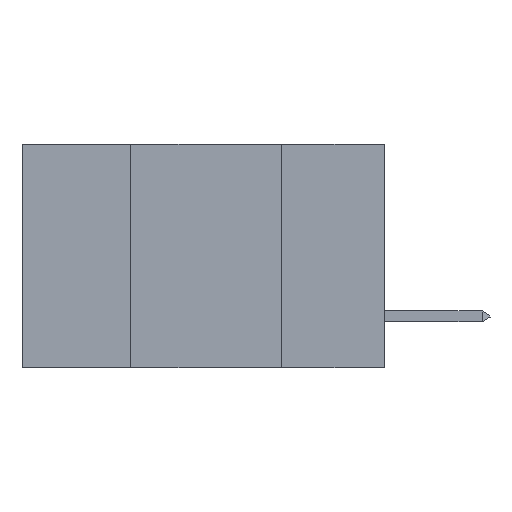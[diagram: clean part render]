
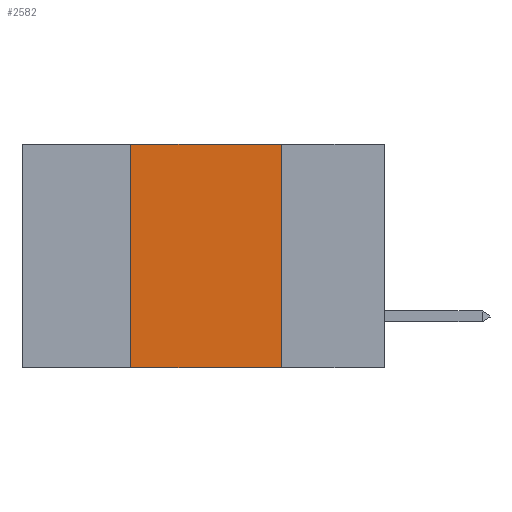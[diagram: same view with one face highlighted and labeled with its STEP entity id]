
A CAD part, left-side view. The second image highlights one B-rep face of the part: STEP entity #2582.
In plain terms, the highlighted planar face has unit normal (-1, 0, 0).
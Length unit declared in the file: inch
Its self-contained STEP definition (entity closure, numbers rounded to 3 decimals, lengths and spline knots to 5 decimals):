
#131 = LINE ( 'NONE', #482, #4072 ) ;
#385 = VERTEX_POINT ( 'NONE', #13871 ) ;
#482 = CARTESIAN_POINT ( 'NONE',  ( 0., 0.6, -0.37 ) ) ;
#1305 = DIRECTION ( 'NONE',  ( 0., -1., 0. ) ) ;
#2582 = ADVANCED_FACE ( 'NONE', ( #24983 ), #10530, .F. ) ;
#3062 = VERTEX_POINT ( 'NONE', #8569 ) ;
#4072 = VECTOR ( 'NONE', #21789, 39.37008 ) ;
#4646 = DIRECTION ( 'NONE',  ( 1., 0., 0. ) ) ;
#4726 = EDGE_CURVE ( 'NONE', #7918, #3062, #7692, .T. ) ;
#6712 = DIRECTION ( 'NONE',  ( 0., 0., -1. ) ) ;
#7692 = LINE ( 'NONE', #21678, #22477 ) ;
#7867 = LINE ( 'NONE', #24668, #24115 ) ;
#7918 = VERTEX_POINT ( 'NONE', #24495 ) ;
#8342 = ORIENTED_EDGE ( 'NONE', *, *, #4726, .F. ) ;
#8569 = CARTESIAN_POINT ( 'NONE',  ( 0., 0.42, 0. ) ) ;
#9111 = VERTEX_POINT ( 'NONE', #10108 ) ;
#10108 = CARTESIAN_POINT ( 'NONE',  ( 0., 0.17, -0.37 ) ) ;
#10530 = PLANE ( 'NONE',  #23315 ) ;
#11037 = VECTOR ( 'NONE', #15741, 39.37008 ) ;
#12194 = DIRECTION ( 'NONE',  ( 0., 0., 1. ) ) ;
#13707 = EDGE_LOOP ( 'NONE', ( #16742, #18024, #8342, #19715 ) ) ;
#13871 = CARTESIAN_POINT ( 'NONE',  ( 0., 0.17, 0. ) ) ;
#14305 = CARTESIAN_POINT ( 'NONE',  ( 0., 0.6, 0. ) ) ;
#15343 = EDGE_CURVE ( 'NONE', #385, #9111, #23066, .T. ) ;
#15741 = DIRECTION ( 'NONE',  ( 0., 0., -1. ) ) ;
#16742 = ORIENTED_EDGE ( 'NONE', *, *, #15343, .F. ) ;
#18024 = ORIENTED_EDGE ( 'NONE', *, *, #18351, .F. ) ;
#18351 = EDGE_CURVE ( 'NONE', #3062, #385, #7867, .T. ) ;
#19690 = CARTESIAN_POINT ( 'NONE',  ( 0., 0.17, 0. ) ) ;
#19715 = ORIENTED_EDGE ( 'NONE', *, *, #20458, .T. ) ;
#20458 = EDGE_CURVE ( 'NONE', #7918, #9111, #131, .T. ) ;
#21678 = CARTESIAN_POINT ( 'NONE',  ( 0., 0.42, 0. ) ) ;
#21789 = DIRECTION ( 'NONE',  ( 0., -1., 0. ) ) ;
#22477 = VECTOR ( 'NONE', #12194, 39.37008 ) ;
#23066 = LINE ( 'NONE', #19690, #11037 ) ;
#23315 = AXIS2_PLACEMENT_3D ( 'NONE', #14305, #4646, #6712 ) ;
#24115 = VECTOR ( 'NONE', #1305, 39.37008 ) ;
#24495 = CARTESIAN_POINT ( 'NONE',  ( 0., 0.42, -0.37 ) ) ;
#24668 = CARTESIAN_POINT ( 'NONE',  ( 0., 0.6, 0. ) ) ;
#24983 = FACE_OUTER_BOUND ( 'NONE', #13707, .T. ) ;
